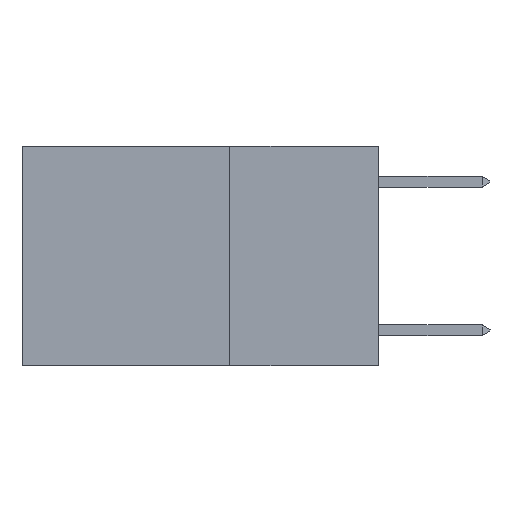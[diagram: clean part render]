
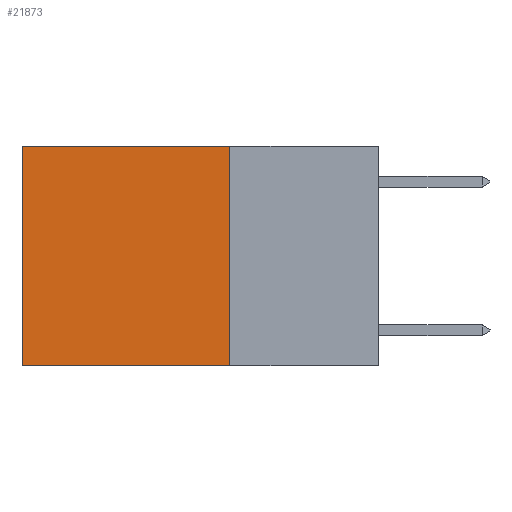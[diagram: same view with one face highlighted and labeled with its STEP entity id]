
A CAD part, left-side view. The second image highlights one B-rep face of the part: STEP entity #21873.
In plain terms, the highlighted planar face has unit normal (-1, 0, 0).
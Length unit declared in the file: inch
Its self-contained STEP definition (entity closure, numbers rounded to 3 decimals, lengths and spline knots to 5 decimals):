
#916 = EDGE_CURVE ( 'NONE', #13592, #8005, #2389, .T. ) ;
#1539 = AXIS2_PLACEMENT_3D ( 'NONE', #22137, #21615, #21593 ) ;
#2268 = ORIENTED_EDGE ( 'NONE', *, *, #15386, .F. ) ;
#2338 = VECTOR ( 'NONE', #9361, 39.37008 ) ;
#2389 = LINE ( 'NONE', #15252, #2338 ) ;
#2989 = CARTESIAN_POINT ( 'NONE',  ( 0.2625, 0.25, -0.37 ) ) ;
#3312 = DIRECTION ( 'NONE',  ( 0., 1., 0. ) ) ;
#3387 = CARTESIAN_POINT ( 'NONE',  ( 0.2625, 0.25, -0.37 ) ) ;
#3697 = VECTOR ( 'NONE', #3312, 39.37008 ) ;
#3759 = LINE ( 'NONE', #3387, #3697 ) ;
#4129 = VECTOR ( 'NONE', #17750, 39.37008 ) ;
#4308 = LINE ( 'NONE', #17253, #4129 ) ;
#5097 = VERTEX_POINT ( 'NONE', #2989 ) ;
#5336 = DIRECTION ( 'NONE',  ( 0., 0., -1. ) ) ;
#5518 = CARTESIAN_POINT ( 'NONE',  ( 0.2625, 0.25, 0. ) ) ;
#8005 = VERTEX_POINT ( 'NONE', #18143 ) ;
#9228 = CARTESIAN_POINT ( 'NONE',  ( 0.2625, 0.25, 0. ) ) ;
#9361 = DIRECTION ( 'NONE',  ( 0., 0., -1. ) ) ;
#12376 = FACE_OUTER_BOUND ( 'NONE', #21482, .T. ) ;
#13407 = ORIENTED_EDGE ( 'NONE', *, *, #21411, .F. ) ;
#13592 = VERTEX_POINT ( 'NONE', #21386 ) ;
#13658 = ORIENTED_EDGE ( 'NONE', *, *, #19589, .T. ) ;
#14766 = VECTOR ( 'NONE', #5336, 39.37008 ) ;
#14874 = LINE ( 'NONE', #5518, #14766 ) ;
#15252 = CARTESIAN_POINT ( 'NONE',  ( 0.2625, 0.6, 0. ) ) ;
#15386 = EDGE_CURVE ( 'NONE', #5097, #8005, #3759, .T. ) ;
#17253 = CARTESIAN_POINT ( 'NONE',  ( 0.2625, 0.25, 0. ) ) ;
#17750 = DIRECTION ( 'NONE',  ( 0., 1., 0. ) ) ;
#18143 = CARTESIAN_POINT ( 'NONE',  ( 0.2625, 0.6, -0.37 ) ) ;
#19589 = EDGE_CURVE ( 'NONE', #21079, #13592, #4308, .T. ) ;
#20483 = ORIENTED_EDGE ( 'NONE', *, *, #916, .T. ) ;
#21079 = VERTEX_POINT ( 'NONE', #9228 ) ;
#21386 = CARTESIAN_POINT ( 'NONE',  ( 0.2625, 0.6, 0. ) ) ;
#21411 = EDGE_CURVE ( 'NONE', #21079, #5097, #14874, .T. ) ;
#21482 = EDGE_LOOP ( 'NONE', ( #20483, #2268, #13407, #13658 ) ) ;
#21593 = DIRECTION ( 'NONE',  ( 0., 0., -1. ) ) ;
#21615 = DIRECTION ( 'NONE',  ( 1., 0., 0. ) ) ;
#21873 = ADVANCED_FACE ( 'NONE', ( #12376 ), #22207, .F. ) ;
#22137 = CARTESIAN_POINT ( 'NONE',  ( 0.2625, 0.25, 0. ) ) ;
#22207 = PLANE ( 'NONE',  #1539 ) ;
